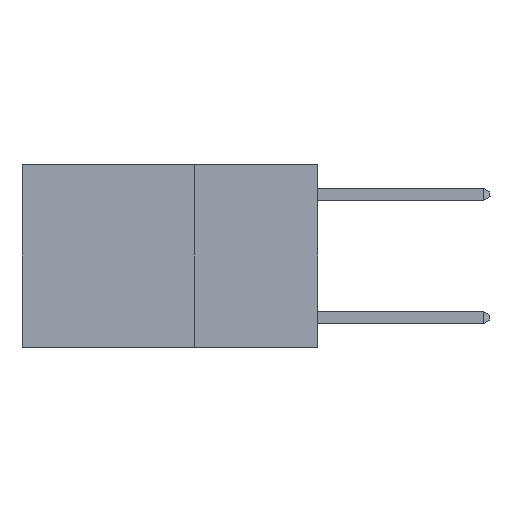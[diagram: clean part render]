
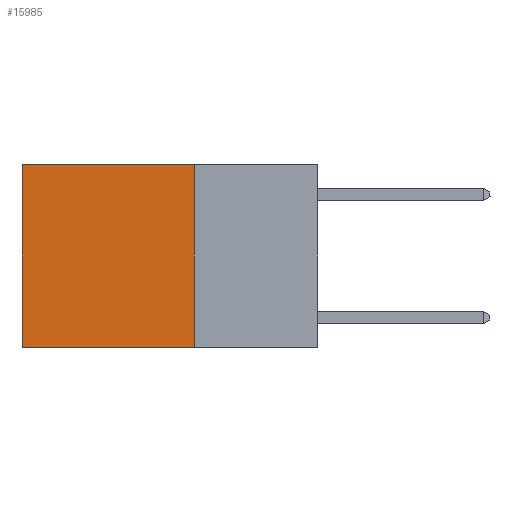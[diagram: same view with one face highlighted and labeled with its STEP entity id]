
A CAD part, left-side view. The second image highlights one B-rep face of the part: STEP entity #15985.
In plain terms, the highlighted planar face has unit normal (-1, 0, 0).
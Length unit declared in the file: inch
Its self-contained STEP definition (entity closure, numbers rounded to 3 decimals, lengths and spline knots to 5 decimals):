
#321 = VERTEX_POINT ( 'NONE', #6956 ) ;
#729 = ORIENTED_EDGE ( 'NONE', *, *, #10817, .F. ) ;
#817 = CARTESIAN_POINT ( 'NONE',  ( 0.2625, 0.6, 0. ) ) ;
#1175 = DIRECTION ( 'NONE',  ( 0., 0., -1. ) ) ;
#2773 = EDGE_LOOP ( 'NONE', ( #4403, #7695, #729, #10253 ) ) ;
#4025 = EDGE_CURVE ( 'NONE', #8067, #6374, #7666, .T. ) ;
#4403 = ORIENTED_EDGE ( 'NONE', *, *, #7731, .T. ) ;
#5866 = VECTOR ( 'NONE', #9174, 39.37008 ) ;
#6374 = VERTEX_POINT ( 'NONE', #9143 ) ;
#6956 = CARTESIAN_POINT ( 'NONE',  ( 0.2625, 0.25, 0. ) ) ;
#7352 = CARTESIAN_POINT ( 'NONE',  ( 0.2625, 0.25, -0.37 ) ) ;
#7515 = CARTESIAN_POINT ( 'NONE',  ( 0.2625, 0.25, 0. ) ) ;
#7666 = LINE ( 'NONE', #7352, #8443 ) ;
#7695 = ORIENTED_EDGE ( 'NONE', *, *, #4025, .F. ) ;
#7731 = EDGE_CURVE ( 'NONE', #18198, #6374, #17288, .T. ) ;
#7838 = LINE ( 'NONE', #7515, #14964 ) ;
#8067 = VERTEX_POINT ( 'NONE', #15816 ) ;
#8114 = EDGE_CURVE ( 'NONE', #321, #18198, #12845, .T. ) ;
#8443 = VECTOR ( 'NONE', #9229, 39.37008 ) ;
#9143 = CARTESIAN_POINT ( 'NONE',  ( 0.2625, 0.6, -0.37 ) ) ;
#9174 = DIRECTION ( 'NONE',  ( 0., 0., -1. ) ) ;
#9229 = DIRECTION ( 'NONE',  ( 0., 1., 0. ) ) ;
#10253 = ORIENTED_EDGE ( 'NONE', *, *, #8114, .T. ) ;
#10348 = VECTOR ( 'NONE', #11099, 39.37008 ) ;
#10817 = EDGE_CURVE ( 'NONE', #321, #8067, #7838, .T. ) ;
#11099 = DIRECTION ( 'NONE',  ( 0., 1., 0. ) ) ;
#11318 = CARTESIAN_POINT ( 'NONE',  ( 0.2625, 0.25, 0. ) ) ;
#12687 = CARTESIAN_POINT ( 'NONE',  ( 0.2625, 0.6, 0. ) ) ;
#12845 = LINE ( 'NONE', #11318, #10348 ) ;
#13026 = PLANE ( 'NONE',  #18260 ) ;
#14964 = VECTOR ( 'NONE', #19570, 39.37008 ) ;
#15816 = CARTESIAN_POINT ( 'NONE',  ( 0.2625, 0.25, -0.37 ) ) ;
#15985 = ADVANCED_FACE ( 'NONE', ( #21349 ), #13026, .F. ) ;
#16206 = DIRECTION ( 'NONE',  ( 1., 0., 0. ) ) ;
#17288 = LINE ( 'NONE', #12687, #5866 ) ;
#18198 = VERTEX_POINT ( 'NONE', #817 ) ;
#18260 = AXIS2_PLACEMENT_3D ( 'NONE', #19694, #16206, #1175 ) ;
#19570 = DIRECTION ( 'NONE',  ( 0., 0., -1. ) ) ;
#19694 = CARTESIAN_POINT ( 'NONE',  ( 0.2625, 0.25, 0. ) ) ;
#21349 = FACE_OUTER_BOUND ( 'NONE', #2773, .T. ) ;
